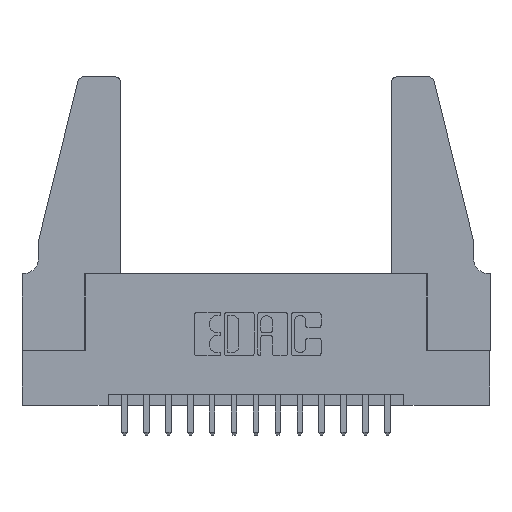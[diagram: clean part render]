
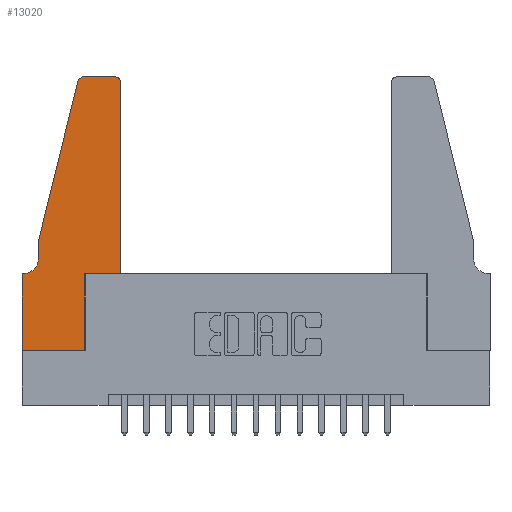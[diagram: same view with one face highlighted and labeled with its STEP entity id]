
A CAD part, top view. The second image highlights one B-rep face of the part: STEP entity #13020.
In plain terms, the highlighted planar face has unit normal (0, 0, 1).
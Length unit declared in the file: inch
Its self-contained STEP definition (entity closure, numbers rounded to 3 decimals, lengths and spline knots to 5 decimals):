
#34 = CARTESIAN_POINT ( 'NONE',  ( 0.0055, 0.35, 0.37 ) ) ;
#53 = CARTESIAN_POINT ( 'NONE',  ( 0., 0., 0.37 ) ) ;
#194 = VERTEX_POINT ( 'NONE', #34 ) ;
#283 = VERTEX_POINT ( 'NONE', #2912 ) ;
#353 = AXIS2_PLACEMENT_3D ( 'NONE', #9569, #1995, #10846 ) ;
#400 = ORIENTED_EDGE ( 'NONE', *, *, #15853, .T. ) ;
#414 = CARTESIAN_POINT ( 'NONE',  ( 0.2605, 1.25, 0.37 ) ) ;
#427 = EDGE_CURVE ( 'NONE', #7010, #13002, #5435, .T. ) ;
#499 = EDGE_CURVE ( 'NONE', #13006, #194, #7612, .T. ) ;
#617 = LINE ( 'NONE', #9184, #13688 ) ;
#1142 = VECTOR ( 'NONE', #6557, 39.37008 ) ;
#1372 = VERTEX_POINT ( 'NONE', #11470 ) ;
#1404 = DIRECTION ( 'NONE',  ( 0., 0., 1. ) ) ;
#1419 = CARTESIAN_POINT ( 'NONE',  ( 0.0755, 0.5, 0.37 ) ) ;
#1530 = AXIS2_PLACEMENT_3D ( 'NONE', #3331, #2147, #7885 ) ;
#1780 = LINE ( 'NONE', #414, #4779 ) ;
#1788 = CARTESIAN_POINT ( 'NONE',  ( 0.0755, 0.42, 0.37 ) ) ;
#1817 = VECTOR ( 'NONE', #7584, 39.37008 ) ;
#1971 = LINE ( 'NONE', #12248, #14983 ) ;
#1995 = DIRECTION ( 'NONE',  ( 0., 0., 1. ) ) ;
#2147 = DIRECTION ( 'NONE',  ( 0., 0., -1. ) ) ;
#2475 = ORIENTED_EDGE ( 'NONE', *, *, #11746, .T. ) ;
#2522 = CARTESIAN_POINT ( 'NONE',  ( 0.2865, 0., 0.37 ) ) ;
#2614 = ORIENTED_EDGE ( 'NONE', *, *, #499, .T. ) ;
#2681 = VERTEX_POINT ( 'NONE', #14077 ) ;
#2912 = CARTESIAN_POINT ( 'NONE',  ( 0.284, 1.25, 0.37 ) ) ;
#3019 = ORIENTED_EDGE ( 'NONE', *, *, #6492, .T. ) ;
#3331 = CARTESIAN_POINT ( 'NONE',  ( 0.0055, 0.42, 0.37 ) ) ;
#3659 = EDGE_CURVE ( 'NONE', #2681, #283, #1780, .T. ) ;
#3858 = EDGE_CURVE ( 'NONE', #4869, #7010, #1971, .T. ) ;
#3965 = ORIENTED_EDGE ( 'NONE', *, *, #3659, .T. ) ;
#4519 = ORIENTED_EDGE ( 'NONE', *, *, #7235, .T. ) ;
#4631 = ORIENTED_EDGE ( 'NONE', *, *, #12730, .T. ) ;
#4706 = DIRECTION ( 'NONE',  ( 1., 0., 0. ) ) ;
#4779 = VECTOR ( 'NONE', #11821, 39.37008 ) ;
#4862 = CARTESIAN_POINT ( 'NONE',  ( 0.0755, 0.5, 0.37 ) ) ;
#4869 = VERTEX_POINT ( 'NONE', #10300 ) ;
#5435 = LINE ( 'NONE', #13808, #8784 ) ;
#5612 = LINE ( 'NONE', #12633, #1817 ) ;
#5631 = PLANE ( 'NONE',  #13324 ) ;
#5671 = CIRCLE ( 'NONE', #353, 0.03 ) ;
#6492 = EDGE_CURVE ( 'NONE', #8648, #13006, #16027, .T. ) ;
#6557 = DIRECTION ( 'NONE',  ( -0.239, -0.971, 0. ) ) ;
#6919 = DIRECTION ( 'NONE',  ( 0., 0., 1. ) ) ;
#7010 = VERTEX_POINT ( 'NONE', #7903 ) ;
#7235 = EDGE_CURVE ( 'NONE', #13002, #2681, #5671, .T. ) ;
#7584 = DIRECTION ( 'NONE',  ( 0., -1., 0. ) ) ;
#7612 = CIRCLE ( 'NONE', #1530, 0.07 ) ;
#7674 = VECTOR ( 'NONE', #9872, 39.37008 ) ;
#7686 = DIRECTION ( 'NONE',  ( 1., 0., 0. ) ) ;
#7885 = DIRECTION ( 'NONE',  ( -1., 0., 0. ) ) ;
#7903 = CARTESIAN_POINT ( 'NONE',  ( 0.4505, 0.35, 0.37 ) ) ;
#8235 = ORIENTED_EDGE ( 'NONE', *, *, #3858, .T. ) ;
#8648 = VERTEX_POINT ( 'NONE', #4862 ) ;
#8736 = VERTEX_POINT ( 'NONE', #2522 ) ;
#8784 = VECTOR ( 'NONE', #11996, 39.37008 ) ;
#8989 = CARTESIAN_POINT ( 'NONE',  ( 0.284, 1.22, 0.37 ) ) ;
#9184 = CARTESIAN_POINT ( 'NONE',  ( 0.2865, 0.35, 0.37 ) ) ;
#9317 = DIRECTION ( 'NONE',  ( 0., -1., 0. ) ) ;
#9569 = CARTESIAN_POINT ( 'NONE',  ( 0.4205, 1.22, 0.37 ) ) ;
#9802 = EDGE_CURVE ( 'NONE', #13268, #8736, #14912, .T. ) ;
#9811 = CARTESIAN_POINT ( 'NONE',  ( 0., 0., 0.37 ) ) ;
#9872 = DIRECTION ( 'NONE',  ( -1., 0., 0. ) ) ;
#9978 = CARTESIAN_POINT ( 'NONE',  ( 0.0755, 0.35, 0.37 ) ) ;
#10272 = DIRECTION ( 'NONE',  ( 1., 0., 0. ) ) ;
#10288 = CARTESIAN_POINT ( 'NONE',  ( 0., 0.35, 0.37 ) ) ;
#10300 = CARTESIAN_POINT ( 'NONE',  ( 0.2865, 0.35, 0.37 ) ) ;
#10590 = ORIENTED_EDGE ( 'NONE', *, *, #9802, .T. ) ;
#10846 = DIRECTION ( 'NONE',  ( 1., 0., 0. ) ) ;
#10984 = VERTEX_POINT ( 'NONE', #10288 ) ;
#11210 = ORIENTED_EDGE ( 'NONE', *, *, #427, .T. ) ;
#11244 = LINE ( 'NONE', #1419, #1142 ) ;
#11470 = CARTESIAN_POINT ( 'NONE',  ( 0.25487, 1.22718, 0.37 ) ) ;
#11746 = EDGE_CURVE ( 'NONE', #8736, #4869, #617, .T. ) ;
#11821 = DIRECTION ( 'NONE',  ( -1., 0., 0. ) ) ;
#11996 = DIRECTION ( 'NONE',  ( 0., 1., 0. ) ) ;
#12248 = CARTESIAN_POINT ( 'NONE',  ( 0.4505, 0.35, 0.37 ) ) ;
#12365 = VECTOR ( 'NONE', #9317, 39.37008 ) ;
#12633 = CARTESIAN_POINT ( 'NONE',  ( 0., 0., 0.37 ) ) ;
#12730 = EDGE_CURVE ( 'NONE', #10984, #13268, #5612, .T. ) ;
#12786 = EDGE_CURVE ( 'NONE', #283, #1372, #14076, .T. ) ;
#12984 = DIRECTION ( 'NONE',  ( 0., 1., 0. ) ) ;
#13002 = VERTEX_POINT ( 'NONE', #15584 ) ;
#13006 = VERTEX_POINT ( 'NONE', #1788 ) ;
#13020 = ADVANCED_FACE ( 'NONE', ( #14647 ), #5631, .T. ) ;
#13268 = VERTEX_POINT ( 'NONE', #9811 ) ;
#13324 = AXIS2_PLACEMENT_3D ( 'NONE', #14421, #6919, #15640 ) ;
#13688 = VECTOR ( 'NONE', #12984, 39.37008 ) ;
#13808 = CARTESIAN_POINT ( 'NONE',  ( 0.4505, 0.35, 0.37 ) ) ;
#13967 = LINE ( 'NONE', #9978, #7674 ) ;
#14076 = CIRCLE ( 'NONE', #14477, 0.03 ) ;
#14077 = CARTESIAN_POINT ( 'NONE',  ( 0.4205, 1.25, 0.37 ) ) ;
#14144 = EDGE_CURVE ( 'NONE', #1372, #8648, #11244, .T. ) ;
#14421 = CARTESIAN_POINT ( 'NONE',  ( 0., 0.35, 0.37 ) ) ;
#14477 = AXIS2_PLACEMENT_3D ( 'NONE', #8989, #1404, #10272 ) ;
#14533 = VECTOR ( 'NONE', #7686, 39.37008 ) ;
#14647 = FACE_OUTER_BOUND ( 'NONE', #16009, .T. ) ;
#14912 = LINE ( 'NONE', #53, #14533 ) ;
#14983 = VECTOR ( 'NONE', #4706, 39.37008 ) ;
#15545 = CARTESIAN_POINT ( 'NONE',  ( 0.0755, 0.5, 0.37 ) ) ;
#15558 = ORIENTED_EDGE ( 'NONE', *, *, #14144, .T. ) ;
#15584 = CARTESIAN_POINT ( 'NONE',  ( 0.4505, 1.22, 0.37 ) ) ;
#15640 = DIRECTION ( 'NONE',  ( 1., 0., 0. ) ) ;
#15853 = EDGE_CURVE ( 'NONE', #194, #10984, #13967, .T. ) ;
#16009 = EDGE_LOOP ( 'NONE', ( #3965, #16095, #15558, #3019, #2614, #400, #4631, #10590, #2475, #8235, #11210, #4519 ) ) ;
#16027 = LINE ( 'NONE', #15545, #12365 ) ;
#16095 = ORIENTED_EDGE ( 'NONE', *, *, #12786, .T. ) ;
